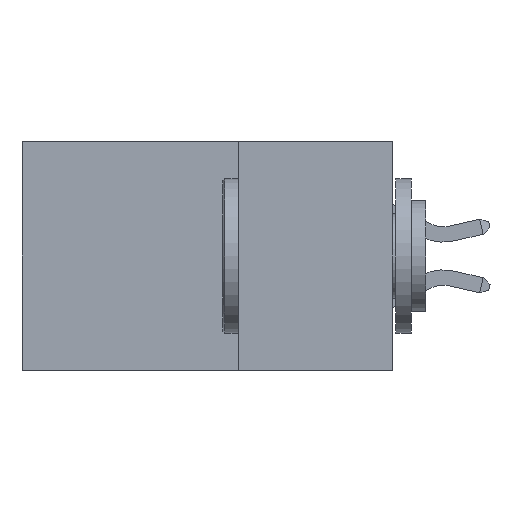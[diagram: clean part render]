
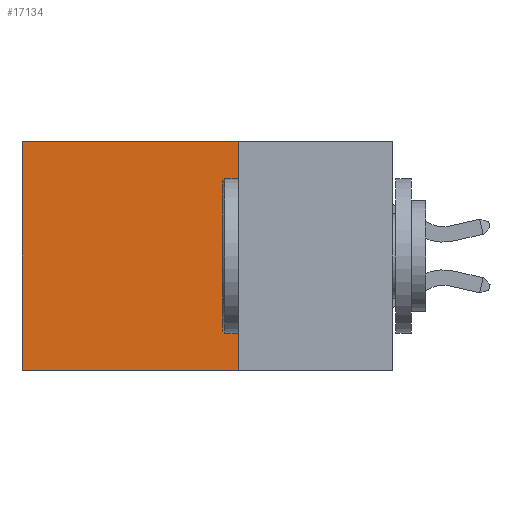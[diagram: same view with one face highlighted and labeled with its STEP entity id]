
A CAD part, left-side view. The second image highlights one B-rep face of the part: STEP entity #17134.
In plain terms, the highlighted planar face has unit normal (-1, 0, 0).
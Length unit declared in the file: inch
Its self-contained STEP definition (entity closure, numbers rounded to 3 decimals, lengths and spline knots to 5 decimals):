
#511 = CARTESIAN_POINT ( 'NONE',  ( 0.2875, 0.6, 0. ) ) ;
#522 = LINE ( 'NONE', #21539, #2745 ) ;
#1295 = VECTOR ( 'NONE', #15733, 39.37008 ) ;
#1963 = CARTESIAN_POINT ( 'NONE',  ( 0.2875, 0.25, -0.37 ) ) ;
#2328 = DIRECTION ( 'NONE',  ( 1., 0., 0. ) ) ;
#2745 = VECTOR ( 'NONE', #17882, 39.37008 ) ;
#3236 = LINE ( 'NONE', #12804, #15075 ) ;
#3354 = CARTESIAN_POINT ( 'NONE',  ( 0.2875, 0.6, 0. ) ) ;
#4068 = EDGE_CURVE ( 'NONE', #10381, #11801, #3236, .T. ) ;
#5221 = EDGE_CURVE ( 'NONE', #19201, #16398, #11421, .T. ) ;
#5347 = CARTESIAN_POINT ( 'NONE',  ( 0.2875, 0.25, 0. ) ) ;
#5705 = ORIENTED_EDGE ( 'NONE', *, *, #4068, .T. ) ;
#5716 = ORIENTED_EDGE ( 'NONE', *, *, #16148, .T. ) ;
#7487 = DIRECTION ( 'NONE',  ( 0., 0., -1. ) ) ;
#8820 = FACE_OUTER_BOUND ( 'NONE', #9280, .T. ) ;
#9280 = EDGE_LOOP ( 'NONE', ( #5716, #10858, #14044, #5705 ) ) ;
#10381 = VERTEX_POINT ( 'NONE', #5347 ) ;
#10858 = ORIENTED_EDGE ( 'NONE', *, *, #5221, .F. ) ;
#11058 = VECTOR ( 'NONE', #21269, 39.37008 ) ;
#11421 = LINE ( 'NONE', #1963, #1295 ) ;
#11801 = VERTEX_POINT ( 'NONE', #511 ) ;
#12804 = CARTESIAN_POINT ( 'NONE',  ( 0.2875, 0.25, 0. ) ) ;
#14044 = ORIENTED_EDGE ( 'NONE', *, *, #20850, .F. ) ;
#14945 = CARTESIAN_POINT ( 'NONE',  ( 0.2875, 0.6, -0.37 ) ) ;
#15075 = VECTOR ( 'NONE', #20186, 39.37008 ) ;
#15311 = CARTESIAN_POINT ( 'NONE',  ( 0.2875, 0.25, -0.37 ) ) ;
#15733 = DIRECTION ( 'NONE',  ( 0., 1., 0. ) ) ;
#16148 = EDGE_CURVE ( 'NONE', #11801, #16398, #22642, .T. ) ;
#16398 = VERTEX_POINT ( 'NONE', #14945 ) ;
#16416 = CARTESIAN_POINT ( 'NONE',  ( 0.2875, 0.25, 0. ) ) ;
#17134 = ADVANCED_FACE ( 'NONE', ( #8820 ), #18056, .F. ) ;
#17882 = DIRECTION ( 'NONE',  ( 0., 0., -1. ) ) ;
#18056 = PLANE ( 'NONE',  #19482 ) ;
#19201 = VERTEX_POINT ( 'NONE', #15311 ) ;
#19482 = AXIS2_PLACEMENT_3D ( 'NONE', #16416, #2328, #7487 ) ;
#20186 = DIRECTION ( 'NONE',  ( 0., 1., 0. ) ) ;
#20850 = EDGE_CURVE ( 'NONE', #10381, #19201, #522, .T. ) ;
#21269 = DIRECTION ( 'NONE',  ( 0., 0., -1. ) ) ;
#21539 = CARTESIAN_POINT ( 'NONE',  ( 0.2875, 0.25, 0. ) ) ;
#22642 = LINE ( 'NONE', #3354, #11058 ) ;
